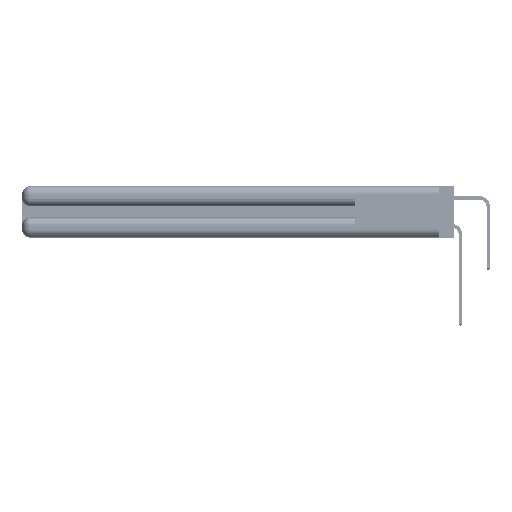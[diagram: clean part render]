
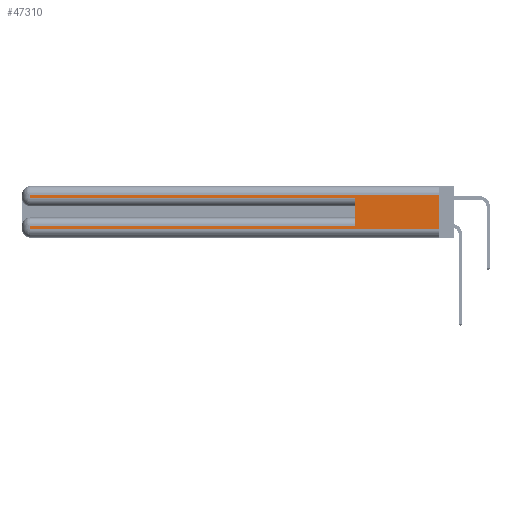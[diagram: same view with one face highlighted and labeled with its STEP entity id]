
A CAD part, left-side view. The second image highlights one B-rep face of the part: STEP entity #47310.
In plain terms, the highlighted planar face has unit normal (-1, 0, 0).
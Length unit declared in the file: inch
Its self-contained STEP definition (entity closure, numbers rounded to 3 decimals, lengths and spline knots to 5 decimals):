
#142 = VERTEX_POINT ( 'NONE', #34065 ) ;
#1995 = VERTEX_POINT ( 'NONE', #19851 ) ;
#2101 = DIRECTION ( 'NONE',  ( 0., 0., -1. ) ) ;
#2472 = CARTESIAN_POINT ( 'NONE',  ( 0., 0., 0.06 ) ) ;
#2869 = FACE_OUTER_BOUND ( 'NONE', #9225, .T. ) ;
#3902 = LINE ( 'NONE', #34430, #48544 ) ;
#6418 = CARTESIAN_POINT ( 'NONE',  ( 0., 0., 0.31 ) ) ;
#8972 = CARTESIAN_POINT ( 'NONE',  ( 0., 0., 0.37 ) ) ;
#9225 = EDGE_LOOP ( 'NONE', ( #44771, #49632, #12684, #21850, #37451, #13924, #53038, #20784 ) ) ;
#12684 = ORIENTED_EDGE ( 'NONE', *, *, #20848, .T. ) ;
#13728 = VECTOR ( 'NONE', #55138, 39.37008 ) ;
#13924 = ORIENTED_EDGE ( 'NONE', *, *, #50062, .T. ) ;
#17303 = EDGE_CURVE ( 'NONE', #55422, #19681, #43876, .T. ) ;
#17457 = VERTEX_POINT ( 'NONE', #44953 ) ;
#18880 = LINE ( 'NONE', #27912, #41863 ) ;
#19436 = VECTOR ( 'NONE', #21804, 39.37008 ) ;
#19681 = VERTEX_POINT ( 'NONE', #58795 ) ;
#19851 = CARTESIAN_POINT ( 'NONE',  ( 0., 0.6, 0.085 ) ) ;
#20029 = DIRECTION ( 'NONE',  ( 0., 0., 1. ) ) ;
#20218 = DIRECTION ( 'NONE',  ( 0., 1., 0. ) ) ;
#20784 = ORIENTED_EDGE ( 'NONE', *, *, #17303, .T. ) ;
#20848 = EDGE_CURVE ( 'NONE', #17457, #44868, #3902, .T. ) ;
#21804 = DIRECTION ( 'NONE',  ( 0., 1., 0. ) ) ;
#21850 = ORIENTED_EDGE ( 'NONE', *, *, #31770, .T. ) ;
#22101 = VECTOR ( 'NONE', #20029, 39.37008 ) ;
#22928 = PLANE ( 'NONE',  #42815 ) ;
#25145 = VERTEX_POINT ( 'NONE', #45603 ) ;
#26012 = LINE ( 'NONE', #49617, #13728 ) ;
#27586 = DIRECTION ( 'NONE',  ( 0., 0., -1. ) ) ;
#27912 = CARTESIAN_POINT ( 'NONE',  ( 0., 0., 0.285 ) ) ;
#30233 = LINE ( 'NONE', #6418, #53048 ) ;
#31631 = CARTESIAN_POINT ( 'NONE',  ( 0., 2.94, 0.285 ) ) ;
#31770 = EDGE_CURVE ( 'NONE', #44868, #142, #18880, .T. ) ;
#31919 = CARTESIAN_POINT ( 'NONE',  ( 0., 2.94, 0.37 ) ) ;
#33955 = EDGE_CURVE ( 'NONE', #45790, #17457, #30233, .T. ) ;
#34065 = CARTESIAN_POINT ( 'NONE',  ( 0., 0.6, 0.285 ) ) ;
#34430 = CARTESIAN_POINT ( 'NONE',  ( 0., 2.94, 0.37 ) ) ;
#37451 = ORIENTED_EDGE ( 'NONE', *, *, #51774, .F. ) ;
#38845 = CARTESIAN_POINT ( 'NONE',  ( 0., 2.94, 0.06 ) ) ;
#39894 = CARTESIAN_POINT ( 'NONE',  ( 0., 0., 0.085 ) ) ;
#41071 = LINE ( 'NONE', #31919, #51742 ) ;
#41412 = EDGE_CURVE ( 'NONE', #25145, #55422, #41071, .T. ) ;
#41863 = VECTOR ( 'NONE', #55202, 39.37008 ) ;
#42457 = VECTOR ( 'NONE', #43779, 39.37008 ) ;
#42815 = AXIS2_PLACEMENT_3D ( 'NONE', #8972, #54874, #27586 ) ;
#42886 = CARTESIAN_POINT ( 'NONE',  ( 0., 0.6, 0.145 ) ) ;
#43779 = DIRECTION ( 'NONE',  ( 0., -1., 0. ) ) ;
#43876 = LINE ( 'NONE', #2472, #42457 ) ;
#44771 = ORIENTED_EDGE ( 'NONE', *, *, #54807, .F. ) ;
#44868 = VERTEX_POINT ( 'NONE', #31631 ) ;
#44953 = CARTESIAN_POINT ( 'NONE',  ( 0., 2.94, 0.31 ) ) ;
#45603 = CARTESIAN_POINT ( 'NONE',  ( 0., 2.94, 0.085 ) ) ;
#45790 = VERTEX_POINT ( 'NONE', #56581 ) ;
#47310 = ADVANCED_FACE ( 'NONE', ( #2869 ), #22928, .F. ) ;
#48544 = VECTOR ( 'NONE', #2101, 39.37008 ) ;
#49617 = CARTESIAN_POINT ( 'NONE',  ( 0., 0., 0.37 ) ) ;
#49632 = ORIENTED_EDGE ( 'NONE', *, *, #33955, .T. ) ;
#50062 = EDGE_CURVE ( 'NONE', #1995, #25145, #57291, .T. ) ;
#50289 = DIRECTION ( 'NONE',  ( 0., 0., -1. ) ) ;
#51742 = VECTOR ( 'NONE', #50289, 39.37008 ) ;
#51774 = EDGE_CURVE ( 'NONE', #1995, #142, #58488, .T. ) ;
#53038 = ORIENTED_EDGE ( 'NONE', *, *, #41412, .T. ) ;
#53048 = VECTOR ( 'NONE', #20218, 39.37008 ) ;
#54807 = EDGE_CURVE ( 'NONE', #45790, #19681, #26012, .T. ) ;
#54874 = DIRECTION ( 'NONE',  ( 1., 0., 0. ) ) ;
#55138 = DIRECTION ( 'NONE',  ( 0., 0., -1. ) ) ;
#55202 = DIRECTION ( 'NONE',  ( 0., -1., 0. ) ) ;
#55422 = VERTEX_POINT ( 'NONE', #38845 ) ;
#56581 = CARTESIAN_POINT ( 'NONE',  ( 0., 0., 0.31 ) ) ;
#57291 = LINE ( 'NONE', #39894, #19436 ) ;
#58488 = LINE ( 'NONE', #42886, #22101 ) ;
#58795 = CARTESIAN_POINT ( 'NONE',  ( 0., 0., 0.06 ) ) ;
